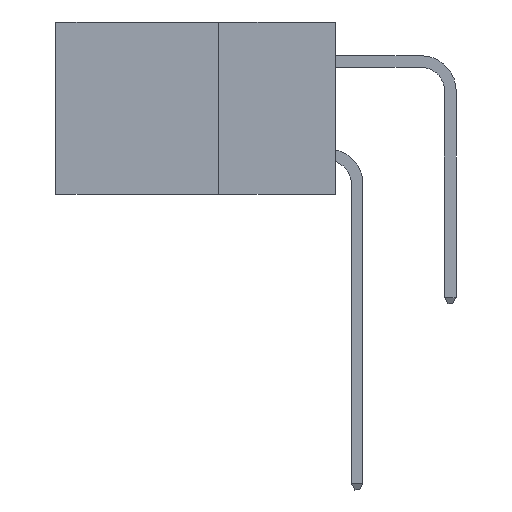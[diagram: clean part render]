
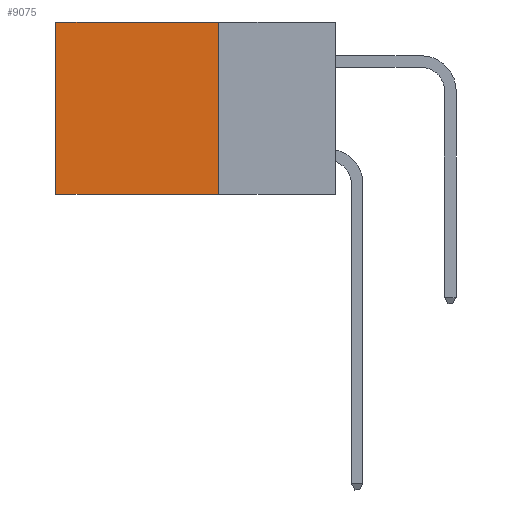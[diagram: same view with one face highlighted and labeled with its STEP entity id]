
A CAD part, left-side view. The second image highlights one B-rep face of the part: STEP entity #9075.
In plain terms, the highlighted planar face has unit normal (-1, 0, 0).
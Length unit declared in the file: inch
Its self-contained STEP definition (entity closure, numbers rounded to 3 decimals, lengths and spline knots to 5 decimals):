
#744 = LINE ( 'NONE', #12724, #4876 ) ;
#1138 = EDGE_CURVE ( 'NONE', #12568, #4941, #7198, .T. ) ;
#1247 = DIRECTION ( 'NONE',  ( 1., 0., 0. ) ) ;
#1704 = VECTOR ( 'NONE', #10889, 39.37008 ) ;
#2213 = EDGE_CURVE ( 'NONE', #11742, #5536, #8577, .T. ) ;
#2393 = DIRECTION ( 'NONE',  ( 0., 0., -1. ) ) ;
#2555 = EDGE_CURVE ( 'NONE', #5536, #4941, #744, .T. ) ;
#3922 = CARTESIAN_POINT ( 'NONE',  ( 0.2875, 0.25, 0. ) ) ;
#4255 = ORIENTED_EDGE ( 'NONE', *, *, #13103, .T. ) ;
#4640 = DIRECTION ( 'NONE',  ( 0., 1., 0. ) ) ;
#4857 = FACE_OUTER_BOUND ( 'NONE', #7911, .T. ) ;
#4876 = VECTOR ( 'NONE', #4640, 39.37008 ) ;
#4941 = VERTEX_POINT ( 'NONE', #5459 ) ;
#5459 = CARTESIAN_POINT ( 'NONE',  ( 0.2875, 0.6, -0.37 ) ) ;
#5536 = VERTEX_POINT ( 'NONE', #5894 ) ;
#5842 = CARTESIAN_POINT ( 'NONE',  ( 0.2875, 0.25, 0. ) ) ;
#5894 = CARTESIAN_POINT ( 'NONE',  ( 0.2875, 0.25, -0.37 ) ) ;
#5946 = ORIENTED_EDGE ( 'NONE', *, *, #2555, .F. ) ;
#6285 = PLANE ( 'NONE',  #10543 ) ;
#6400 = DIRECTION ( 'NONE',  ( 0., 0., -1. ) ) ;
#7198 = LINE ( 'NONE', #10532, #12774 ) ;
#7468 = CARTESIAN_POINT ( 'NONE',  ( 0.2875, 0.6, 0. ) ) ;
#7911 = EDGE_LOOP ( 'NONE', ( #12775, #5946, #11220, #4255 ) ) ;
#8400 = VECTOR ( 'NONE', #6400, 39.37008 ) ;
#8577 = LINE ( 'NONE', #12339, #8400 ) ;
#8814 = DIRECTION ( 'NONE',  ( 0., 0., -1. ) ) ;
#9075 = ADVANCED_FACE ( 'NONE', ( #4857 ), #6285, .F. ) ;
#10532 = CARTESIAN_POINT ( 'NONE',  ( 0.2875, 0.6, 0. ) ) ;
#10543 = AXIS2_PLACEMENT_3D ( 'NONE', #12384, #1247, #2393 ) ;
#10889 = DIRECTION ( 'NONE',  ( 0., 1., 0. ) ) ;
#11220 = ORIENTED_EDGE ( 'NONE', *, *, #2213, .F. ) ;
#11742 = VERTEX_POINT ( 'NONE', #3922 ) ;
#12339 = CARTESIAN_POINT ( 'NONE',  ( 0.2875, 0.25, 0. ) ) ;
#12384 = CARTESIAN_POINT ( 'NONE',  ( 0.2875, 0.25, 0. ) ) ;
#12530 = LINE ( 'NONE', #5842, #1704 ) ;
#12568 = VERTEX_POINT ( 'NONE', #7468 ) ;
#12724 = CARTESIAN_POINT ( 'NONE',  ( 0.2875, 0.25, -0.37 ) ) ;
#12774 = VECTOR ( 'NONE', #8814, 39.37008 ) ;
#12775 = ORIENTED_EDGE ( 'NONE', *, *, #1138, .T. ) ;
#13103 = EDGE_CURVE ( 'NONE', #11742, #12568, #12530, .T. ) ;
